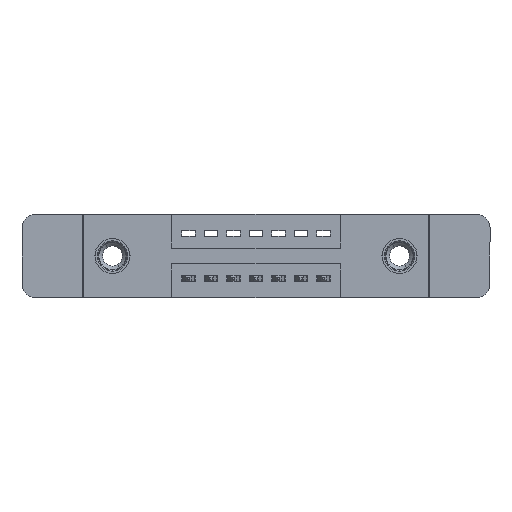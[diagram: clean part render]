
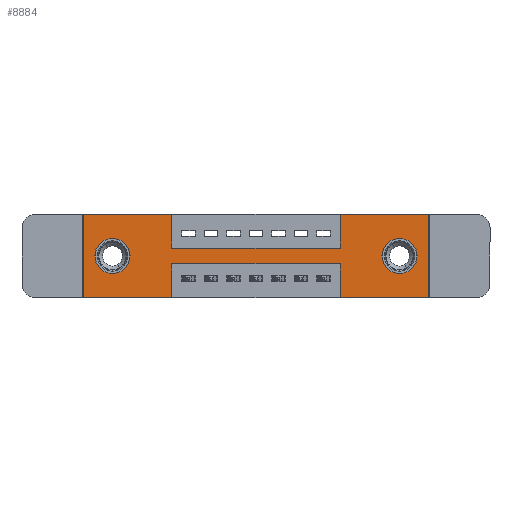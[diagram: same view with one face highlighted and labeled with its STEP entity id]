
A CAD part, front view. The second image highlights one B-rep face of the part: STEP entity #8884.
In plain terms, the highlighted planar face has unit normal (0, -1, 0).
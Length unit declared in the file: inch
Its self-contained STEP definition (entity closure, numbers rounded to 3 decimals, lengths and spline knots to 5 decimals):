
#11 = LINE ( 'NONE', #1846, #14500 ) ;
#59 = CARTESIAN_POINT ( 'NONE',  ( 0.13, 0., -0.107 ) ) ;
#64 = CARTESIAN_POINT ( 'NONE',  ( 0., 0., 0. ) ) ;
#82 = VERTEX_POINT ( 'NONE', #7035 ) ;
#95 = ORIENTED_EDGE ( 'NONE', *, *, #2291, .F. ) ;
#160 = ORIENTED_EDGE ( 'NONE', *, *, #13553, .T. ) ;
#345 = DIRECTION ( 'NONE',  ( 0., -1., 0. ) ) ;
#393 = CARTESIAN_POINT ( 'NONE',  ( 0., 0., -0.37 ) ) ;
#470 = VERTEX_POINT ( 'NONE', #3924 ) ;
#528 = EDGE_LOOP ( 'NONE', ( #7167, #1789, #12184, #10758, #6043, #3022, #13513, #3058, #12905, #13010, #95, #8715 ) ) ;
#534 = AXIS2_PLACEMENT_3D ( 'NONE', #9192, #7881, #9144 ) ;
#646 = CARTESIAN_POINT ( 'NONE',  ( 0.13, 0., -0.263 ) ) ;
#670 = CARTESIAN_POINT ( 'NONE',  ( 0.3925, 0., -0.22 ) ) ;
#1016 = VECTOR ( 'NONE', #9552, 39.37008 ) ;
#1103 = VERTEX_POINT ( 'NONE', #14765 ) ;
#1144 = EDGE_CURVE ( 'NONE', #2673, #11303, #11764, .T. ) ;
#1187 = ORIENTED_EDGE ( 'NONE', *, *, #9618, .T. ) ;
#1216 = VERTEX_POINT ( 'NONE', #5584 ) ;
#1336 = LINE ( 'NONE', #7008, #8476 ) ;
#1412 = DIRECTION ( 'NONE',  ( 1., 0., 0. ) ) ;
#1504 = VECTOR ( 'NONE', #2055, 39.37008 ) ;
#1593 = DIRECTION ( 'NONE',  ( 0., 0., -1. ) ) ;
#1789 = ORIENTED_EDGE ( 'NONE', *, *, #14693, .F. ) ;
#1846 = CARTESIAN_POINT ( 'NONE',  ( 1.535, 0., 0. ) ) ;
#2055 = DIRECTION ( 'NONE',  ( 0., 0., 1. ) ) ;
#2169 = CARTESIAN_POINT ( 'NONE',  ( 1.1425, 0., 0. ) ) ;
#2291 = EDGE_CURVE ( 'NONE', #8720, #6343, #3858, .T. ) ;
#2347 = CARTESIAN_POINT ( 'NONE',  ( 0., 0., -0.37 ) ) ;
#2393 = CARTESIAN_POINT ( 'NONE',  ( 0., 0., 0. ) ) ;
#2488 = CARTESIAN_POINT ( 'NONE',  ( 1.405, 0., -0.185 ) ) ;
#2597 = CARTESIAN_POINT ( 'NONE',  ( 0., 0., -0.37 ) ) ;
#2673 = VERTEX_POINT ( 'NONE', #5299 ) ;
#2736 = DIRECTION ( 'NONE',  ( 0., 0., -1. ) ) ;
#2927 = CARTESIAN_POINT ( 'NONE',  ( 0., 0., 0. ) ) ;
#3022 = ORIENTED_EDGE ( 'NONE', *, *, #12472, .F. ) ;
#3058 = ORIENTED_EDGE ( 'NONE', *, *, #11439, .F. ) ;
#3123 = VECTOR ( 'NONE', #9668, 39.37008 ) ;
#3179 = LINE ( 'NONE', #8676, #6279 ) ;
#3381 = DIRECTION ( 'NONE',  ( 0., 0., 1. ) ) ;
#3858 = LINE ( 'NONE', #2393, #11913 ) ;
#3867 = AXIS2_PLACEMENT_3D ( 'NONE', #393, #345, #8599 ) ;
#3924 = CARTESIAN_POINT ( 'NONE',  ( 0.3925, 0., -0.22 ) ) ;
#4077 = VERTEX_POINT ( 'NONE', #8835 ) ;
#4094 = PLANE ( 'NONE',  #3867 ) ;
#4175 = AXIS2_PLACEMENT_3D ( 'NONE', #9684, #9851, #1593 ) ;
#4301 = VERTEX_POINT ( 'NONE', #8427 ) ;
#4383 = CARTESIAN_POINT ( 'NONE',  ( 1.535, 0., -0.37 ) ) ;
#5184 = CARTESIAN_POINT ( 'NONE',  ( 1.1425, 0., -0.37 ) ) ;
#5265 = EDGE_CURVE ( 'NONE', #9593, #4301, #9339, .T. ) ;
#5299 = CARTESIAN_POINT ( 'NONE',  ( 1.1425, 0., -0.15 ) ) ;
#5369 = DIRECTION ( 'NONE',  ( -1., 0., 0. ) ) ;
#5584 = CARTESIAN_POINT ( 'NONE',  ( 1.535, 0., 0. ) ) ;
#5760 = FACE_BOUND ( 'NONE', #7219, .T. ) ;
#5970 = CARTESIAN_POINT ( 'NONE',  ( 0.3925, 0., -0.37 ) ) ;
#6043 = ORIENTED_EDGE ( 'NONE', *, *, #14672, .F. ) ;
#6174 = CARTESIAN_POINT ( 'NONE',  ( 1.405, 0., -0.263 ) ) ;
#6279 = VECTOR ( 'NONE', #2736, 39.37008 ) ;
#6298 = AXIS2_PLACEMENT_3D ( 'NONE', #7055, #10513, #3381 ) ;
#6343 = VERTEX_POINT ( 'NONE', #14619 ) ;
#6459 = CARTESIAN_POINT ( 'NONE',  ( 0., 0., -0.37 ) ) ;
#6659 = VECTOR ( 'NONE', #11124, 39.37008 ) ;
#6800 = CARTESIAN_POINT ( 'NONE',  ( 1.1425, 0., 0. ) ) ;
#7008 = CARTESIAN_POINT ( 'NONE',  ( 0.3925, 0., 0. ) ) ;
#7035 = CARTESIAN_POINT ( 'NONE',  ( 0.3925, 0., 0. ) ) ;
#7055 = CARTESIAN_POINT ( 'NONE',  ( 0.13, 0., -0.185 ) ) ;
#7111 = VECTOR ( 'NONE', #8315, 39.37008 ) ;
#7167 = ORIENTED_EDGE ( 'NONE', *, *, #13643, .F. ) ;
#7219 = EDGE_LOOP ( 'NONE', ( #1187, #160 ) ) ;
#7338 = DIRECTION ( 'NONE',  ( 0., 1., 0. ) ) ;
#7551 = VECTOR ( 'NONE', #5369, 39.37008 ) ;
#7787 = CIRCLE ( 'NONE', #534, 0.078 ) ;
#7870 = LINE ( 'NONE', #6459, #7111 ) ;
#7881 = DIRECTION ( 'NONE',  ( 0., 1., 0. ) ) ;
#8294 = EDGE_CURVE ( 'NONE', #13812, #9491, #9826, .T. ) ;
#8315 = DIRECTION ( 'NONE',  ( -1., 0., 0. ) ) ;
#8427 = CARTESIAN_POINT ( 'NONE',  ( 1.1425, 0., -0.22 ) ) ;
#8476 = VECTOR ( 'NONE', #10709, 39.37008 ) ;
#8599 = DIRECTION ( 'NONE',  ( 0., 0., -1. ) ) ;
#8673 = CIRCLE ( 'NONE', #14952, 0.078 ) ;
#8676 = CARTESIAN_POINT ( 'NONE',  ( 0.3925, 0., -0.37 ) ) ;
#8715 = ORIENTED_EDGE ( 'NONE', *, *, #11643, .F. ) ;
#8720 = VERTEX_POINT ( 'NONE', #2347 ) ;
#8745 = VERTEX_POINT ( 'NONE', #5970 ) ;
#8835 = CARTESIAN_POINT ( 'NONE',  ( 1.405, 0., -0.107 ) ) ;
#8884 = ADVANCED_FACE ( 'NONE', ( #5760, #11635, #9612 ), #4094, .T. ) ;
#8931 = DIRECTION ( 'NONE',  ( 1., 0., 0. ) ) ;
#9047 = LINE ( 'NONE', #2927, #6659 ) ;
#9144 = DIRECTION ( 'NONE',  ( 0., 0., 1. ) ) ;
#9192 = CARTESIAN_POINT ( 'NONE',  ( 0.13, 0., -0.185 ) ) ;
#9266 = ORIENTED_EDGE ( 'NONE', *, *, #8294, .T. ) ;
#9339 = LINE ( 'NONE', #14313, #3123 ) ;
#9376 = EDGE_LOOP ( 'NONE', ( #13076, #9266 ) ) ;
#9410 = EDGE_CURVE ( 'NONE', #13750, #9593, #7870, .T. ) ;
#9491 = VERTEX_POINT ( 'NONE', #59 ) ;
#9535 = DIRECTION ( 'NONE',  ( 0., 0., -1. ) ) ;
#9552 = DIRECTION ( 'NONE',  ( -1., 0., 0. ) ) ;
#9593 = VERTEX_POINT ( 'NONE', #5184 ) ;
#9612 = FACE_OUTER_BOUND ( 'NONE', #528, .T. ) ;
#9618 = EDGE_CURVE ( 'NONE', #4077, #14442, #11160, .T. ) ;
#9668 = DIRECTION ( 'NONE',  ( 0., 0., 1. ) ) ;
#9684 = CARTESIAN_POINT ( 'NONE',  ( 1.405, 0., -0.185 ) ) ;
#9826 = CIRCLE ( 'NONE', #6298, 0.078 ) ;
#9851 = DIRECTION ( 'NONE',  ( 0., 1., 0. ) ) ;
#10045 = DIRECTION ( 'NONE',  ( 0., 0., -1. ) ) ;
#10177 = CARTESIAN_POINT ( 'NONE',  ( 0.3925, 0., -0.15 ) ) ;
#10188 = LINE ( 'NONE', #2597, #1016 ) ;
#10410 = EDGE_CURVE ( 'NONE', #6343, #82, #14994, .T. ) ;
#10513 = DIRECTION ( 'NONE',  ( 0., 1., 0. ) ) ;
#10691 = DIRECTION ( 'NONE',  ( 0., 0., 1. ) ) ;
#10709 = DIRECTION ( 'NONE',  ( 0., 0., -1. ) ) ;
#10758 = ORIENTED_EDGE ( 'NONE', *, *, #9410, .F. ) ;
#11124 = DIRECTION ( 'NONE',  ( 1., 0., 0. ) ) ;
#11160 = CIRCLE ( 'NONE', #4175, 0.078 ) ;
#11283 = LINE ( 'NONE', #10177, #13668 ) ;
#11303 = VERTEX_POINT ( 'NONE', #2169 ) ;
#11439 = EDGE_CURVE ( 'NONE', #1103, #2673, #11283, .T. ) ;
#11635 = FACE_BOUND ( 'NONE', #9376, .T. ) ;
#11643 = EDGE_CURVE ( 'NONE', #8745, #8720, #10188, .T. ) ;
#11764 = LINE ( 'NONE', #6800, #1504 ) ;
#11913 = VECTOR ( 'NONE', #10691, 39.37008 ) ;
#12184 = ORIENTED_EDGE ( 'NONE', *, *, #5265, .F. ) ;
#12472 = EDGE_CURVE ( 'NONE', #11303, #1216, #9047, .T. ) ;
#12905 = ORIENTED_EDGE ( 'NONE', *, *, #14033, .F. ) ;
#13010 = ORIENTED_EDGE ( 'NONE', *, *, #10410, .F. ) ;
#13076 = ORIENTED_EDGE ( 'NONE', *, *, #13337, .T. ) ;
#13337 = EDGE_CURVE ( 'NONE', #9491, #13812, #7787, .T. ) ;
#13513 = ORIENTED_EDGE ( 'NONE', *, *, #1144, .F. ) ;
#13553 = EDGE_CURVE ( 'NONE', #14442, #4077, #8673, .T. ) ;
#13643 = EDGE_CURVE ( 'NONE', #470, #8745, #3179, .T. ) ;
#13668 = VECTOR ( 'NONE', #8931, 39.37008 ) ;
#13698 = VECTOR ( 'NONE', #1412, 39.37008 ) ;
#13750 = VERTEX_POINT ( 'NONE', #4383 ) ;
#13812 = VERTEX_POINT ( 'NONE', #646 ) ;
#14033 = EDGE_CURVE ( 'NONE', #82, #1103, #1336, .T. ) ;
#14313 = CARTESIAN_POINT ( 'NONE',  ( 1.1425, 0., -0.37 ) ) ;
#14442 = VERTEX_POINT ( 'NONE', #6174 ) ;
#14500 = VECTOR ( 'NONE', #10045, 39.37008 ) ;
#14619 = CARTESIAN_POINT ( 'NONE',  ( 0., 0., 0. ) ) ;
#14672 = EDGE_CURVE ( 'NONE', #1216, #13750, #11, .T. ) ;
#14693 = EDGE_CURVE ( 'NONE', #4301, #470, #15049, .T. ) ;
#14765 = CARTESIAN_POINT ( 'NONE',  ( 0.3925, 0., -0.15 ) ) ;
#14952 = AXIS2_PLACEMENT_3D ( 'NONE', #2488, #7338, #9535 ) ;
#14994 = LINE ( 'NONE', #64, #13698 ) ;
#15049 = LINE ( 'NONE', #670, #7551 ) ;
